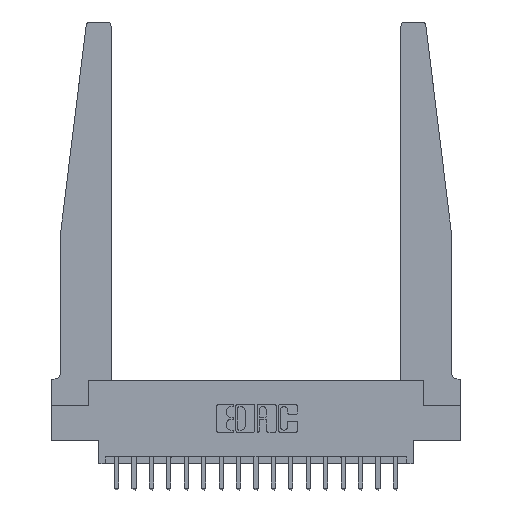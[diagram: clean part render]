
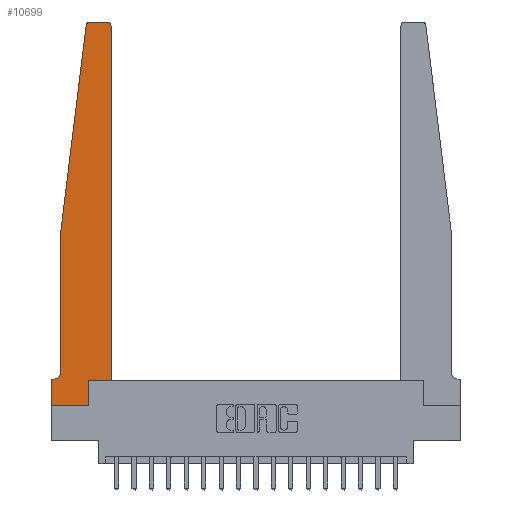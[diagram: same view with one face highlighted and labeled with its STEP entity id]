
A CAD part, top view. The second image highlights one B-rep face of the part: STEP entity #10699.
In plain terms, the highlighted planar face has unit normal (0, 0, 1).
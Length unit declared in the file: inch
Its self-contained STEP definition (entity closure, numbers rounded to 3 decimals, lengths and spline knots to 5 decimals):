
#42 = ORIENTED_EDGE ( 'NONE', *, *, #16794, .T. ) ;
#408 = ORIENTED_EDGE ( 'NONE', *, *, #10005, .T. ) ;
#759 = VECTOR ( 'NONE', #13104, 39.37008 ) ;
#980 = VECTOR ( 'NONE', #6351, 39.37008 ) ;
#1414 = ORIENTED_EDGE ( 'NONE', *, *, #2098, .T. ) ;
#1438 = EDGE_CURVE ( 'NONE', #17717, #12113, #7154, .T. ) ;
#1764 = ORIENTED_EDGE ( 'NONE', *, *, #5231, .T. ) ;
#2087 = CARTESIAN_POINT ( 'NONE',  ( 0.2605, 0.18, 0.37 ) ) ;
#2098 = EDGE_CURVE ( 'NONE', #13629, #10883, #13177, .T. ) ;
#2186 = DIRECTION ( 'NONE',  ( 0., 1., 0. ) ) ;
#3098 = EDGE_LOOP ( 'NONE', ( #16903, #1414, #14733, #11151, #42, #1764, #17980, #19071, #3607, #17069, #408, #7821 ) ) ;
#3149 = EDGE_CURVE ( 'NONE', #10883, #17840, #4807, .T. ) ;
#3309 = CARTESIAN_POINT ( 'NONE',  ( 0.2605, 0.18, 0.37 ) ) ;
#3520 = CARTESIAN_POINT ( 'NONE',  ( 0.24675, 2.72367, 0.37 ) ) ;
#3607 = ORIENTED_EDGE ( 'NONE', *, *, #5555, .T. ) ;
#3902 = CARTESIAN_POINT ( 'NONE',  ( 0.015, 0.1875, 0.37 ) ) ;
#4270 = AXIS2_PLACEMENT_3D ( 'NONE', #6451, #4743, #9469 ) ;
#4715 = DIRECTION ( 'NONE',  ( 0., 1., 0. ) ) ;
#4743 = DIRECTION ( 'NONE',  ( 0., 0., 1. ) ) ;
#4807 = LINE ( 'NONE', #12155, #7685 ) ;
#4813 = EDGE_CURVE ( 'NONE', #16606, #13629, #9174, .T. ) ;
#5231 = EDGE_CURVE ( 'NONE', #8639, #7904, #10557, .T. ) ;
#5555 = EDGE_CURVE ( 'NONE', #19745, #17717, #9835, .T. ) ;
#5793 = DIRECTION ( 'NONE',  ( -1., 0., 0. ) ) ;
#5869 = AXIS2_PLACEMENT_3D ( 'NONE', #10869, #6344, #18345 ) ;
#6063 = AXIS2_PLACEMENT_3D ( 'NONE', #9899, #8489, #8588 ) ;
#6344 = DIRECTION ( 'NONE',  ( 0., 0., 1. ) ) ;
#6351 = DIRECTION ( 'NONE',  ( -1., 0., 0. ) ) ;
#6362 = VERTEX_POINT ( 'NONE', #7645 ) ;
#6451 = CARTESIAN_POINT ( 'NONE',  ( 0., 0.1875, 0.37 ) ) ;
#6970 = CARTESIAN_POINT ( 'NONE',  ( 0., 0., 0.37 ) ) ;
#7154 = LINE ( 'NONE', #13380, #14452 ) ;
#7645 = CARTESIAN_POINT ( 'NONE',  ( 0.065, 0.2375, 0.37 ) ) ;
#7685 = VECTOR ( 'NONE', #9526, 39.37008 ) ;
#7821 = ORIENTED_EDGE ( 'NONE', *, *, #9570, .T. ) ;
#7904 = VERTEX_POINT ( 'NONE', #10589 ) ;
#8489 = DIRECTION ( 'NONE',  ( 0., 0., 1. ) ) ;
#8575 = CARTESIAN_POINT ( 'NONE',  ( 0.2605, 0., 0.37 ) ) ;
#8588 = DIRECTION ( 'NONE',  ( 1., 0., 0. ) ) ;
#8639 = VERTEX_POINT ( 'NONE', #3902 ) ;
#9174 = LINE ( 'NONE', #10972, #980 ) ;
#9216 = EDGE_CURVE ( 'NONE', #19454, #19745, #12819, .T. ) ;
#9469 = DIRECTION ( 'NONE',  ( 1., 0., 0. ) ) ;
#9526 = DIRECTION ( 'NONE',  ( -0.122, -0.992, 0. ) ) ;
#9570 = EDGE_CURVE ( 'NONE', #15672, #16606, #17114, .T. ) ;
#9605 = DIRECTION ( 'NONE',  ( 0., -1., 0. ) ) ;
#9835 = LINE ( 'NONE', #2087, #16742 ) ;
#9899 = CARTESIAN_POINT ( 'NONE',  ( 0.27653, 2.72, 0.37 ) ) ;
#10005 = EDGE_CURVE ( 'NONE', #12113, #15672, #13474, .T. ) ;
#10042 = CARTESIAN_POINT ( 'NONE',  ( 0., 0., 0.37 ) ) ;
#10440 = CARTESIAN_POINT ( 'NONE',  ( 0.425, 0.18, 0.37 ) ) ;
#10446 = CIRCLE ( 'NONE', #12050, 0.05 ) ;
#10557 = LINE ( 'NONE', #12170, #17709 ) ;
#10589 = CARTESIAN_POINT ( 'NONE',  ( 0., 0.1875, 0.37 ) ) ;
#10671 = CARTESIAN_POINT ( 'NONE',  ( 0.065, 1.25, 0.37 ) ) ;
#10699 = ADVANCED_FACE ( 'NONE', ( #19752 ), #18543, .T. ) ;
#10869 = CARTESIAN_POINT ( 'NONE',  ( 0.395, 2.72, 0.37 ) ) ;
#10883 = VERTEX_POINT ( 'NONE', #3520 ) ;
#10972 = CARTESIAN_POINT ( 'NONE',  ( 0.25, 2.75, 0.37 ) ) ;
#11151 = ORIENTED_EDGE ( 'NONE', *, *, #16893, .T. ) ;
#11851 = LINE ( 'NONE', #10042, #16283 ) ;
#11963 = DIRECTION ( 'NONE',  ( 1., 0., 0. ) ) ;
#12050 = AXIS2_PLACEMENT_3D ( 'NONE', #16755, #16365, #5793 ) ;
#12113 = VERTEX_POINT ( 'NONE', #10440 ) ;
#12155 = CARTESIAN_POINT ( 'NONE',  ( 0.065, 1.25, 0.37 ) ) ;
#12170 = CARTESIAN_POINT ( 'NONE',  ( 0.065, 0.1875, 0.37 ) ) ;
#12320 = VECTOR ( 'NONE', #4715, 39.37008 ) ;
#12819 = LINE ( 'NONE', #6970, #759 ) ;
#13104 = DIRECTION ( 'NONE',  ( 1., 0., 0. ) ) ;
#13177 = CIRCLE ( 'NONE', #6063, 0.03 ) ;
#13380 = CARTESIAN_POINT ( 'NONE',  ( 0.425, 0.18, 0.37 ) ) ;
#13474 = LINE ( 'NONE', #18514, #12320 ) ;
#13629 = VERTEX_POINT ( 'NONE', #19490 ) ;
#13682 = VECTOR ( 'NONE', #9605, 39.37008 ) ;
#13939 = CARTESIAN_POINT ( 'NONE',  ( 0.065, 1.25, 0.37 ) ) ;
#14452 = VECTOR ( 'NONE', #11963, 39.37008 ) ;
#14491 = EDGE_CURVE ( 'NONE', #7904, #19454, #11851, .T. ) ;
#14733 = ORIENTED_EDGE ( 'NONE', *, *, #3149, .T. ) ;
#15031 = CARTESIAN_POINT ( 'NONE',  ( 0.425, 2.72, 0.37 ) ) ;
#15672 = VERTEX_POINT ( 'NONE', #15031 ) ;
#15980 = CARTESIAN_POINT ( 'NONE',  ( 0., 0., 0.37 ) ) ;
#16283 = VECTOR ( 'NONE', #19326, 39.37008 ) ;
#16365 = DIRECTION ( 'NONE',  ( 0., 0., -1. ) ) ;
#16606 = VERTEX_POINT ( 'NONE', #19202 ) ;
#16742 = VECTOR ( 'NONE', #2186, 39.37008 ) ;
#16755 = CARTESIAN_POINT ( 'NONE',  ( 0.015, 0.2375, 0.37 ) ) ;
#16794 = EDGE_CURVE ( 'NONE', #6362, #8639, #10446, .T. ) ;
#16893 = EDGE_CURVE ( 'NONE', #17840, #6362, #18482, .T. ) ;
#16903 = ORIENTED_EDGE ( 'NONE', *, *, #4813, .T. ) ;
#17069 = ORIENTED_EDGE ( 'NONE', *, *, #1438, .T. ) ;
#17114 = CIRCLE ( 'NONE', #5869, 0.03 ) ;
#17709 = VECTOR ( 'NONE', #19728, 39.37008 ) ;
#17717 = VERTEX_POINT ( 'NONE', #3309 ) ;
#17840 = VERTEX_POINT ( 'NONE', #10671 ) ;
#17980 = ORIENTED_EDGE ( 'NONE', *, *, #14491, .T. ) ;
#18345 = DIRECTION ( 'NONE',  ( 1., 0., 0. ) ) ;
#18482 = LINE ( 'NONE', #13939, #13682 ) ;
#18514 = CARTESIAN_POINT ( 'NONE',  ( 0.425, 0.18, 0.37 ) ) ;
#18543 = PLANE ( 'NONE',  #4270 ) ;
#19071 = ORIENTED_EDGE ( 'NONE', *, *, #9216, .T. ) ;
#19202 = CARTESIAN_POINT ( 'NONE',  ( 0.395, 2.75, 0.37 ) ) ;
#19326 = DIRECTION ( 'NONE',  ( 0., -1., 0. ) ) ;
#19454 = VERTEX_POINT ( 'NONE', #15980 ) ;
#19490 = CARTESIAN_POINT ( 'NONE',  ( 0.27653, 2.75, 0.37 ) ) ;
#19728 = DIRECTION ( 'NONE',  ( -1., 0., 0. ) ) ;
#19745 = VERTEX_POINT ( 'NONE', #8575 ) ;
#19752 = FACE_OUTER_BOUND ( 'NONE', #3098, .T. ) ;
